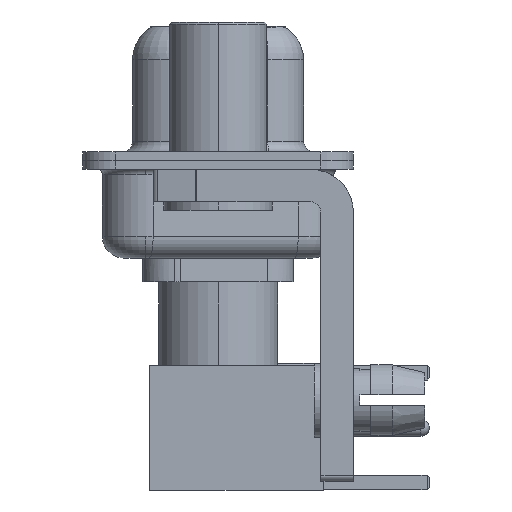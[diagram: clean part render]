
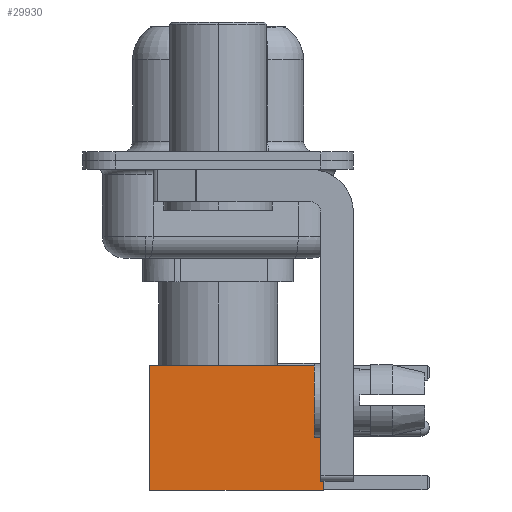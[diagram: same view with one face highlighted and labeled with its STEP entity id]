
A CAD part, left-side view. The second image highlights one B-rep face of the part: STEP entity #29930.
In plain terms, the highlighted face is planar.
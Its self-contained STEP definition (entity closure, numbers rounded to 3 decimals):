
#1122 = CARTESIAN_POINT ( 'NONE',  ( 2.875, 2.875, 8. ) ) ;
#1624 = EDGE_CURVE ( 'NONE', #18877, #29687, #30937, .T. ) ;
#1830 = DIRECTION ( 'NONE',  ( 0., 0., -1. ) ) ;
#4181 = ORIENTED_EDGE ( 'NONE', *, *, #1624, .T. ) ;
#4235 = CARTESIAN_POINT ( 'NONE',  ( 2.875, 2.875, 0. ) ) ;
#4386 = VERTEX_POINT ( 'NONE', #18991 ) ;
#4622 = FACE_OUTER_BOUND ( 'NONE', #21827, .T. ) ;
#4937 = PLANE ( 'NONE',  #20152 ) ;
#5001 = ORIENTED_EDGE ( 'NONE', *, *, #17135, .T. ) ;
#5473 = LINE ( 'NONE', #27665, #25124 ) ;
#7220 = VECTOR ( 'NONE', #11480, 1000. ) ;
#8811 = VECTOR ( 'NONE', #1830, 1000. ) ;
#9435 = CARTESIAN_POINT ( 'NONE',  ( 2.875, 2.875, 0. ) ) ;
#11097 = ORIENTED_EDGE ( 'NONE', *, *, #23117, .F. ) ;
#11480 = DIRECTION ( 'NONE',  ( 0., 0., -1. ) ) ;
#11684 = DIRECTION ( 'NONE',  ( -1., 0., 0. ) ) ;
#11844 = CARTESIAN_POINT ( 'NONE',  ( 0., 2.875, 0. ) ) ;
#11951 = CARTESIAN_POINT ( 'NONE',  ( -2.875, 2.875, 0. ) ) ;
#15698 = CARTESIAN_POINT ( 'NONE',  ( -2.875, 2.875, 8. ) ) ;
#16224 = LINE ( 'NONE', #11844, #30130 ) ;
#17135 = EDGE_CURVE ( 'NONE', #29687, #4386, #16224, .T. ) ;
#18877 = VERTEX_POINT ( 'NONE', #1122 ) ;
#18991 = CARTESIAN_POINT ( 'NONE',  ( -2.875, 2.875, 0. ) ) ;
#19291 = DIRECTION ( 'NONE',  ( 0., 1., 0. ) ) ;
#19602 = DIRECTION ( 'NONE',  ( 0., 0., 1. ) ) ;
#20152 = AXIS2_PLACEMENT_3D ( 'NONE', #9435, #19291, #19602 ) ;
#21827 = EDGE_LOOP ( 'NONE', ( #4181, #5001, #11097, #27960 ) ) ;
#22665 = CARTESIAN_POINT ( 'NONE',  ( 2.875, 2.875, 0. ) ) ;
#22986 = VERTEX_POINT ( 'NONE', #15698 ) ;
#23117 = EDGE_CURVE ( 'NONE', #22986, #4386, #23398, .T. ) ;
#23398 = LINE ( 'NONE', #11951, #7220 ) ;
#25124 = VECTOR ( 'NONE', #30232, 1000. ) ;
#25850 = EDGE_CURVE ( 'NONE', #18877, #22986, #5473, .T. ) ;
#27665 = CARTESIAN_POINT ( 'NONE',  ( 0., 2.875, 8. ) ) ;
#27960 = ORIENTED_EDGE ( 'NONE', *, *, #25850, .F. ) ;
#29687 = VERTEX_POINT ( 'NONE', #22665 ) ;
#29930 = ADVANCED_FACE ( 'NONE', ( #4622 ), #4937, .T. ) ;
#30130 = VECTOR ( 'NONE', #11684, 1000. ) ;
#30232 = DIRECTION ( 'NONE',  ( -1., 0., 0. ) ) ;
#30937 = LINE ( 'NONE', #4235, #8811 ) ;
